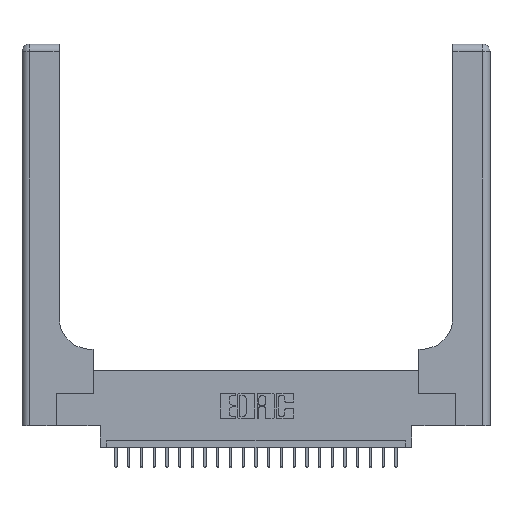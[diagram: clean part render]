
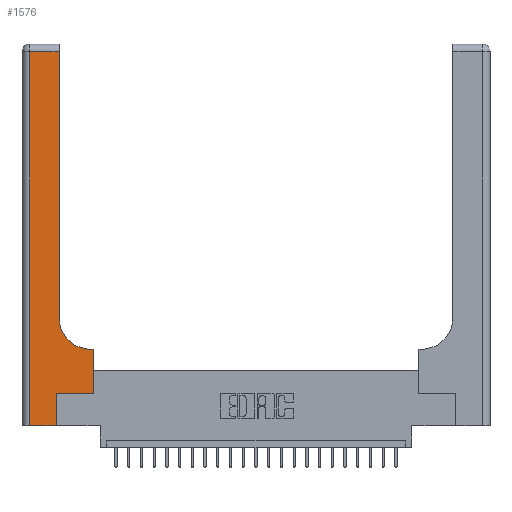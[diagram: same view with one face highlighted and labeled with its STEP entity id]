
A CAD part, top view. The second image highlights one B-rep face of the part: STEP entity #1576.
In plain terms, the highlighted planar face has unit normal (0, 0, 1).
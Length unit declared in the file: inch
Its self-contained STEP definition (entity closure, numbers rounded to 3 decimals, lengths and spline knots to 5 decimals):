
#262 = CARTESIAN_POINT ( 'NONE',  ( 0.5585, 0.6, 0.37 ) ) ;
#604 = CARTESIAN_POINT ( 'NONE',  ( 0.5415, 0.85, 0.37 ) ) ;
#614 = LINE ( 'NONE', #11299, #21714 ) ;
#640 = DIRECTION ( 'NONE',  ( 0., 1., 0. ) ) ;
#717 = DIRECTION ( 'NONE',  ( 1., 0., 0. ) ) ;
#785 = ORIENTED_EDGE ( 'NONE', *, *, #1022, .T. ) ;
#942 = AXIS2_PLACEMENT_3D ( 'NONE', #604, #10172, #2548 ) ;
#1022 = EDGE_CURVE ( 'NONE', #9923, #5921, #1680, .T. ) ;
#1576 = ADVANCED_FACE ( 'NONE', ( #22788 ), #2493, .F. ) ;
#1680 = LINE ( 'NONE', #14241, #14544 ) ;
#2327 = CARTESIAN_POINT ( 'NONE',  ( 0.2915, 2.94, 0.37 ) ) ;
#2466 = EDGE_CURVE ( 'NONE', #16177, #9923, #17491, .T. ) ;
#2493 = PLANE ( 'NONE',  #5007 ) ;
#2548 = DIRECTION ( 'NONE',  ( 1., 0., 0. ) ) ;
#2714 = EDGE_CURVE ( 'NONE', #7105, #7892, #22988, .T. ) ;
#3003 = VECTOR ( 'NONE', #8363, 39.37008 ) ;
#3040 = CARTESIAN_POINT ( 'NONE',  ( 0.2915, 0.85, 0.37 ) ) ;
#3115 = VERTEX_POINT ( 'NONE', #2327 ) ;
#3612 = CARTESIAN_POINT ( 'NONE',  ( 0.06, 2.94, 0.37 ) ) ;
#3793 = DIRECTION ( 'NONE',  ( -1., 0., 0. ) ) ;
#3804 = CARTESIAN_POINT ( 'NONE',  ( 0.5415, 0.6, 0.37 ) ) ;
#4177 = LINE ( 'NONE', #12024, #3003 ) ;
#4788 = EDGE_CURVE ( 'NONE', #22293, #16805, #9727, .T. ) ;
#5007 = AXIS2_PLACEMENT_3D ( 'NONE', #10118, #10375, #23789 ) ;
#5278 = EDGE_CURVE ( 'NONE', #16805, #9327, #22853, .T. ) ;
#5921 = VERTEX_POINT ( 'NONE', #262 ) ;
#6452 = CARTESIAN_POINT ( 'NONE',  ( 0.06, 0., 0.37 ) ) ;
#6948 = CARTESIAN_POINT ( 'NONE',  ( 0.5585, 0.25, 0.37 ) ) ;
#7065 = EDGE_LOOP ( 'NONE', ( #24372, #18022, #12725, #7497, #16739, #9567, #785, #24067, #22943 ) ) ;
#7105 = VERTEX_POINT ( 'NONE', #3804 ) ;
#7212 = DIRECTION ( 'NONE',  ( 0., -1., 0. ) ) ;
#7497 = ORIENTED_EDGE ( 'NONE', *, *, #5278, .T. ) ;
#7806 = LINE ( 'NONE', #23208, #24906 ) ;
#7892 = VERTEX_POINT ( 'NONE', #3040 ) ;
#8363 = DIRECTION ( 'NONE',  ( 0., 1., 0. ) ) ;
#9327 = VERTEX_POINT ( 'NONE', #22458 ) ;
#9567 = ORIENTED_EDGE ( 'NONE', *, *, #2466, .T. ) ;
#9727 = LINE ( 'NONE', #20239, #10341 ) ;
#9734 = VECTOR ( 'NONE', #19045, 39.37008 ) ;
#9923 = VERTEX_POINT ( 'NONE', #6948 ) ;
#10118 = CARTESIAN_POINT ( 'NONE',  ( 0., 3., 0.37 ) ) ;
#10172 = DIRECTION ( 'NONE',  ( 0., 0., -1. ) ) ;
#10341 = VECTOR ( 'NONE', #7212, 39.37008 ) ;
#10375 = DIRECTION ( 'NONE',  ( 0., 0., -1. ) ) ;
#11299 = CARTESIAN_POINT ( 'NONE',  ( 0.2915, 3., 0.37 ) ) ;
#12024 = CARTESIAN_POINT ( 'NONE',  ( 0.269, 0., 0.37 ) ) ;
#12169 = EDGE_CURVE ( 'NONE', #7892, #3115, #614, .T. ) ;
#12725 = ORIENTED_EDGE ( 'NONE', *, *, #4788, .T. ) ;
#12856 = EDGE_CURVE ( 'NONE', #3115, #22293, #15857, .T. ) ;
#13470 = CARTESIAN_POINT ( 'NONE',  ( 0., 2.94, 0.37 ) ) ;
#14241 = CARTESIAN_POINT ( 'NONE',  ( 0.5585, 0.25, 0.37 ) ) ;
#14332 = EDGE_CURVE ( 'NONE', #5921, #7105, #7806, .T. ) ;
#14544 = VECTOR ( 'NONE', #640, 39.37008 ) ;
#15857 = LINE ( 'NONE', #13470, #9734 ) ;
#16177 = VERTEX_POINT ( 'NONE', #23059 ) ;
#16739 = ORIENTED_EDGE ( 'NONE', *, *, #21444, .T. ) ;
#16805 = VERTEX_POINT ( 'NONE', #6452 ) ;
#17241 = DIRECTION ( 'NONE',  ( 1., 0., 0. ) ) ;
#17491 = LINE ( 'NONE', #21932, #18715 ) ;
#18022 = ORIENTED_EDGE ( 'NONE', *, *, #12856, .T. ) ;
#18715 = VECTOR ( 'NONE', #717, 39.37008 ) ;
#19045 = DIRECTION ( 'NONE',  ( -1., 0., 0. ) ) ;
#20239 = CARTESIAN_POINT ( 'NONE',  ( 0.06, 3., 0.37 ) ) ;
#20424 = VECTOR ( 'NONE', #17241, 39.37008 ) ;
#20873 = DIRECTION ( 'NONE',  ( 0., 1., 0. ) ) ;
#21444 = EDGE_CURVE ( 'NONE', #9327, #16177, #4177, .T. ) ;
#21714 = VECTOR ( 'NONE', #20873, 39.37008 ) ;
#21932 = CARTESIAN_POINT ( 'NONE',  ( 0.269, 0.25, 0.37 ) ) ;
#22293 = VERTEX_POINT ( 'NONE', #3612 ) ;
#22458 = CARTESIAN_POINT ( 'NONE',  ( 0.269, 0., 0.37 ) ) ;
#22788 = FACE_OUTER_BOUND ( 'NONE', #7065, .T. ) ;
#22853 = LINE ( 'NONE', #25064, #20424 ) ;
#22943 = ORIENTED_EDGE ( 'NONE', *, *, #2714, .T. ) ;
#22988 = CIRCLE ( 'NONE', #942, 0.25 ) ;
#23059 = CARTESIAN_POINT ( 'NONE',  ( 0.269, 0.25, 0.37 ) ) ;
#23208 = CARTESIAN_POINT ( 'NONE',  ( 0.2915, 0.6, 0.37 ) ) ;
#23789 = DIRECTION ( 'NONE',  ( -1., 0., 0. ) ) ;
#24067 = ORIENTED_EDGE ( 'NONE', *, *, #14332, .T. ) ;
#24372 = ORIENTED_EDGE ( 'NONE', *, *, #12169, .T. ) ;
#24906 = VECTOR ( 'NONE', #3793, 39.37008 ) ;
#25064 = CARTESIAN_POINT ( 'NONE',  ( 0., 0., 0.37 ) ) ;
